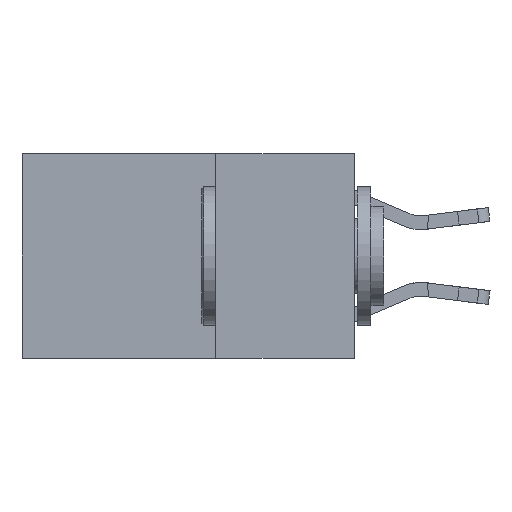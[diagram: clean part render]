
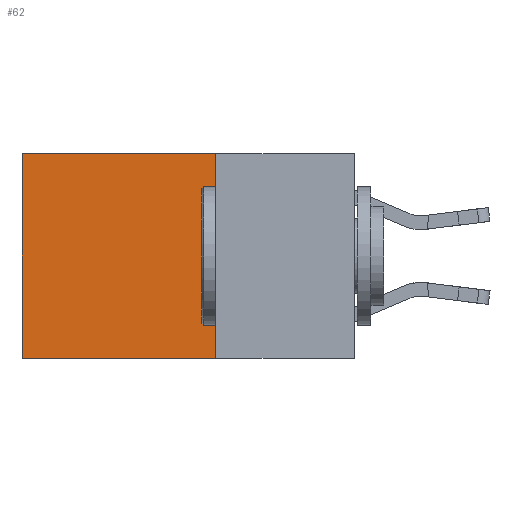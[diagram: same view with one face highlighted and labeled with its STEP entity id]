
A CAD part, left-side view. The second image highlights one B-rep face of the part: STEP entity #62.
In plain terms, the highlighted planar face has unit normal (-1, 0, 0).
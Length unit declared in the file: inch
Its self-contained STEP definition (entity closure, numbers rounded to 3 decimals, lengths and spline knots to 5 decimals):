
#62 = ADVANCED_FACE ( 'NONE', ( #16054 ), #19021, .F. ) ;
#378 = VECTOR ( 'NONE', #10965, 39.37008 ) ;
#1839 = VERTEX_POINT ( 'NONE', #21535 ) ;
#3142 = CARTESIAN_POINT ( 'NONE',  ( 0.2625, 0.6, 0. ) ) ;
#3648 = LINE ( 'NONE', #18363, #13883 ) ;
#4286 = ORIENTED_EDGE ( 'NONE', *, *, #5998, .T. ) ;
#5457 = AXIS2_PLACEMENT_3D ( 'NONE', #6842, #8936, #23061 ) ;
#5998 = EDGE_CURVE ( 'NONE', #24384, #11414, #16248, .T. ) ;
#6636 = DIRECTION ( 'NONE',  ( 0., 0., -1. ) ) ;
#6842 = CARTESIAN_POINT ( 'NONE',  ( 0.2625, 0.25, 0. ) ) ;
#7190 = CARTESIAN_POINT ( 'NONE',  ( 0.2625, 0.25, -0.37 ) ) ;
#8936 = DIRECTION ( 'NONE',  ( 1., 0., 0. ) ) ;
#9361 = CARTESIAN_POINT ( 'NONE',  ( 0.2625, 0.25, 0. ) ) ;
#9445 = DIRECTION ( 'NONE',  ( 0., 1., 0. ) ) ;
#10208 = VECTOR ( 'NONE', #9445, 39.37008 ) ;
#10965 = DIRECTION ( 'NONE',  ( 0., 0., -1. ) ) ;
#11414 = VERTEX_POINT ( 'NONE', #3142 ) ;
#11637 = CARTESIAN_POINT ( 'NONE',  ( 0.2625, 0.25, 0. ) ) ;
#11702 = EDGE_CURVE ( 'NONE', #23434, #1839, #3648, .T. ) ;
#12615 = ORIENTED_EDGE ( 'NONE', *, *, #18415, .T. ) ;
#13006 = VECTOR ( 'NONE', #6636, 39.37008 ) ;
#13623 = LINE ( 'NONE', #14752, #13006 ) ;
#13883 = VECTOR ( 'NONE', #20397, 39.37008 ) ;
#14752 = CARTESIAN_POINT ( 'NONE',  ( 0.2625, 0.25, 0. ) ) ;
#15507 = EDGE_LOOP ( 'NONE', ( #12615, #23959, #19871, #4286 ) ) ;
#16054 = FACE_OUTER_BOUND ( 'NONE', #15507, .T. ) ;
#16098 = LINE ( 'NONE', #23033, #378 ) ;
#16248 = LINE ( 'NONE', #9361, #10208 ) ;
#17158 = EDGE_CURVE ( 'NONE', #24384, #23434, #13623, .T. ) ;
#18363 = CARTESIAN_POINT ( 'NONE',  ( 0.2625, 0.25, -0.37 ) ) ;
#18415 = EDGE_CURVE ( 'NONE', #11414, #1839, #16098, .T. ) ;
#19021 = PLANE ( 'NONE',  #5457 ) ;
#19871 = ORIENTED_EDGE ( 'NONE', *, *, #17158, .F. ) ;
#20397 = DIRECTION ( 'NONE',  ( 0., 1., 0. ) ) ;
#21535 = CARTESIAN_POINT ( 'NONE',  ( 0.2625, 0.6, -0.37 ) ) ;
#23033 = CARTESIAN_POINT ( 'NONE',  ( 0.2625, 0.6, 0. ) ) ;
#23061 = DIRECTION ( 'NONE',  ( 0., 0., -1. ) ) ;
#23434 = VERTEX_POINT ( 'NONE', #7190 ) ;
#23959 = ORIENTED_EDGE ( 'NONE', *, *, #11702, .F. ) ;
#24384 = VERTEX_POINT ( 'NONE', #11637 ) ;
